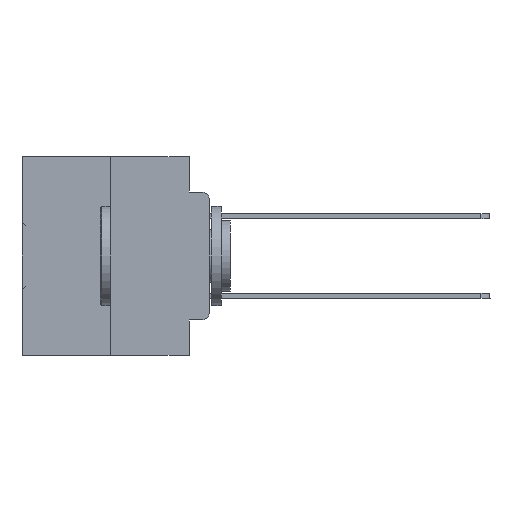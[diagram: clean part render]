
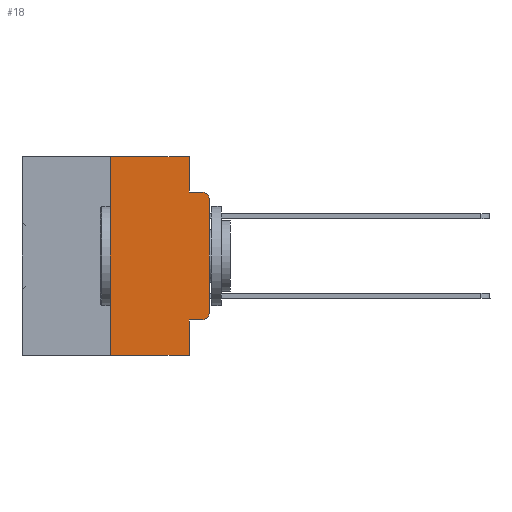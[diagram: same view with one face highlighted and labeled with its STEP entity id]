
A CAD part, left-side view. The second image highlights one B-rep face of the part: STEP entity #18.
In plain terms, the highlighted planar face has unit normal (-1, 0, 0).
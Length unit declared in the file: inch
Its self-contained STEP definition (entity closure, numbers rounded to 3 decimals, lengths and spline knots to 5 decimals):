
#18 = ADVANCED_FACE ( 'NONE', ( #32277 ), #12737, .F. ) ;
#543 = CARTESIAN_POINT ( 'NONE',  ( 0., 0.051, -0.0885 ) ) ;
#781 = LINE ( 'NONE', #25487, #34024 ) ;
#959 = CARTESIAN_POINT ( 'NONE',  ( 0., 0.051, -0.4115 ) ) ;
#1598 = VERTEX_POINT ( 'NONE', #15078 ) ;
#1759 = DIRECTION ( 'NONE',  ( 0., 0., -1. ) ) ;
#2859 = VECTOR ( 'NONE', #4577, 39.37008 ) ;
#3428 = CARTESIAN_POINT ( 'NONE',  ( 0., 0., 0. ) ) ;
#3833 = VERTEX_POINT ( 'NONE', #23011 ) ;
#3874 = VERTEX_POINT ( 'NONE', #543 ) ;
#3929 = DIRECTION ( 'NONE',  ( 0., 0., -1. ) ) ;
#4577 = DIRECTION ( 'NONE',  ( 0., -1., 0. ) ) ;
#4684 = DIRECTION ( 'NONE',  ( -1., 0., 0. ) ) ;
#4919 = VECTOR ( 'NONE', #28663, 39.37008 ) ;
#5046 = CIRCLE ( 'NONE', #35947, 0.02 ) ;
#5157 = LINE ( 'NONE', #29843, #15808 ) ;
#5775 = DIRECTION ( 'NONE',  ( 0., 0., -1. ) ) ;
#6001 = LINE ( 'NONE', #3428, #4919 ) ;
#6632 = DIRECTION ( 'NONE',  ( 0., -1., 0. ) ) ;
#6854 = CARTESIAN_POINT ( 'NONE',  ( 0., 0.02, -0.1085 ) ) ;
#7220 = CARTESIAN_POINT ( 'NONE',  ( 0., 0.02, -0.0885 ) ) ;
#7312 = CIRCLE ( 'NONE', #29499, 0.02 ) ;
#7621 = CARTESIAN_POINT ( 'NONE',  ( 0., 0.02, -0.4115 ) ) ;
#8134 = VERTEX_POINT ( 'NONE', #15001 ) ;
#8910 = ORIENTED_EDGE ( 'NONE', *, *, #16786, .F. ) ;
#9737 = CARTESIAN_POINT ( 'NONE',  ( 0., 0.25, 0. ) ) ;
#10545 = CARTESIAN_POINT ( 'NONE',  ( 0., 0.02, -0.3915 ) ) ;
#11173 = EDGE_CURVE ( 'NONE', #1598, #12328, #20268, .T. ) ;
#11231 = EDGE_CURVE ( 'NONE', #23768, #34738, #6001, .T. ) ;
#11914 = VECTOR ( 'NONE', #31216, 39.37008 ) ;
#12090 = ORIENTED_EDGE ( 'NONE', *, *, #14174, .T. ) ;
#12142 = DIRECTION ( 'NONE',  ( 0., 0., -1. ) ) ;
#12328 = VERTEX_POINT ( 'NONE', #9737 ) ;
#12737 = PLANE ( 'NONE',  #20117 ) ;
#13576 = DIRECTION ( 'NONE',  ( 0., -1., 0. ) ) ;
#14174 = EDGE_CURVE ( 'NONE', #34738, #28405, #7312, .T. ) ;
#15001 = CARTESIAN_POINT ( 'NONE',  ( 0., 0.051, -0.4115 ) ) ;
#15078 = CARTESIAN_POINT ( 'NONE',  ( 0., 0.25, -0.5 ) ) ;
#15808 = VECTOR ( 'NONE', #13576, 39.37008 ) ;
#16760 = CARTESIAN_POINT ( 'NONE',  ( 0., 0.051, 0. ) ) ;
#16786 = EDGE_CURVE ( 'NONE', #12328, #3833, #781, .T. ) ;
#17270 = CARTESIAN_POINT ( 'NONE',  ( 0., 0.051, 0. ) ) ;
#18471 = CARTESIAN_POINT ( 'NONE',  ( 0., 0.051, -0.0885 ) ) ;
#19632 = VECTOR ( 'NONE', #12142, 39.37008 ) ;
#20117 = AXIS2_PLACEMENT_3D ( 'NONE', #23481, #24217, #3929 ) ;
#20268 = LINE ( 'NONE', #28837, #11914 ) ;
#21125 = EDGE_CURVE ( 'NONE', #26871, #23768, #5046, .T. ) ;
#21310 = ORIENTED_EDGE ( 'NONE', *, *, #24610, .F. ) ;
#21448 = EDGE_CURVE ( 'NONE', #3833, #3874, #28421, .T. ) ;
#23011 = CARTESIAN_POINT ( 'NONE',  ( 0., 0.051, 0. ) ) ;
#23064 = LINE ( 'NONE', #959, #23146 ) ;
#23146 = VECTOR ( 'NONE', #6632, 39.37008 ) ;
#23375 = CARTESIAN_POINT ( 'NONE',  ( 0., 0., -0.3915 ) ) ;
#23481 = CARTESIAN_POINT ( 'NONE',  ( 0., 0.473, 0. ) ) ;
#23612 = ORIENTED_EDGE ( 'NONE', *, *, #21448, .F. ) ;
#23768 = VERTEX_POINT ( 'NONE', #23375 ) ;
#23850 = ORIENTED_EDGE ( 'NONE', *, *, #25959, .F. ) ;
#24117 = VERTEX_POINT ( 'NONE', #25032 ) ;
#24217 = DIRECTION ( 'NONE',  ( 1., 0., 0. ) ) ;
#24260 = EDGE_LOOP ( 'NONE', ( #31616, #12090, #23850, #23612, #8910, #25479, #28085, #21310, #27536, #30254 ) ) ;
#24610 = EDGE_CURVE ( 'NONE', #8134, #24117, #28436, .T. ) ;
#25032 = CARTESIAN_POINT ( 'NONE',  ( 0., 0.051, -0.5 ) ) ;
#25479 = ORIENTED_EDGE ( 'NONE', *, *, #11173, .F. ) ;
#25487 = CARTESIAN_POINT ( 'NONE',  ( 0., 0.473, 0. ) ) ;
#25959 = EDGE_CURVE ( 'NONE', #3874, #28405, #32724, .T. ) ;
#26871 = VERTEX_POINT ( 'NONE', #7621 ) ;
#27536 = ORIENTED_EDGE ( 'NONE', *, *, #30094, .T. ) ;
#28085 = ORIENTED_EDGE ( 'NONE', *, *, #34768, .T. ) ;
#28405 = VERTEX_POINT ( 'NONE', #7220 ) ;
#28421 = LINE ( 'NONE', #17270, #19632 ) ;
#28436 = LINE ( 'NONE', #16760, #32069 ) ;
#28663 = DIRECTION ( 'NONE',  ( 0., 0., 1. ) ) ;
#28837 = CARTESIAN_POINT ( 'NONE',  ( 0., 0.25, 0. ) ) ;
#28947 = DIRECTION ( 'NONE',  ( 0., -1., 0. ) ) ;
#29169 = DIRECTION ( 'NONE',  ( 0., 0., -1. ) ) ;
#29499 = AXIS2_PLACEMENT_3D ( 'NONE', #6854, #34618, #29169 ) ;
#29843 = CARTESIAN_POINT ( 'NONE',  ( 0., 0.473, -0.5 ) ) ;
#30094 = EDGE_CURVE ( 'NONE', #8134, #26871, #23064, .T. ) ;
#30254 = ORIENTED_EDGE ( 'NONE', *, *, #21125, .T. ) ;
#31216 = DIRECTION ( 'NONE',  ( 0., 0., 1. ) ) ;
#31616 = ORIENTED_EDGE ( 'NONE', *, *, #11231, .T. ) ;
#32069 = VECTOR ( 'NONE', #5775, 39.37008 ) ;
#32277 = FACE_OUTER_BOUND ( 'NONE', #24260, .T. ) ;
#32724 = LINE ( 'NONE', #18471, #2859 ) ;
#33127 = CARTESIAN_POINT ( 'NONE',  ( 0., 0., -0.1085 ) ) ;
#34024 = VECTOR ( 'NONE', #28947, 39.37008 ) ;
#34618 = DIRECTION ( 'NONE',  ( -1., 0., 0. ) ) ;
#34738 = VERTEX_POINT ( 'NONE', #33127 ) ;
#34768 = EDGE_CURVE ( 'NONE', #1598, #24117, #5157, .T. ) ;
#35947 = AXIS2_PLACEMENT_3D ( 'NONE', #10545, #4684, #1759 ) ;
